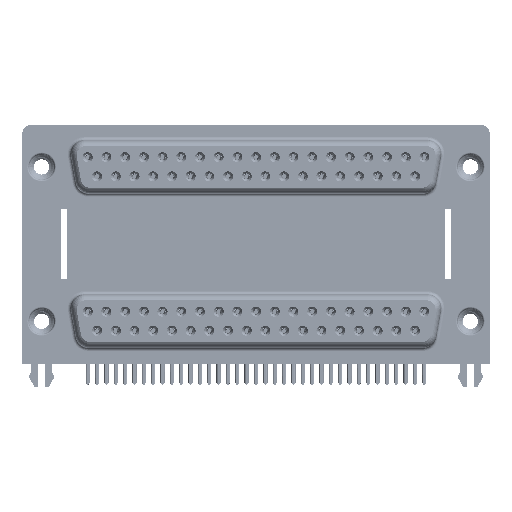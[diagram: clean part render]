
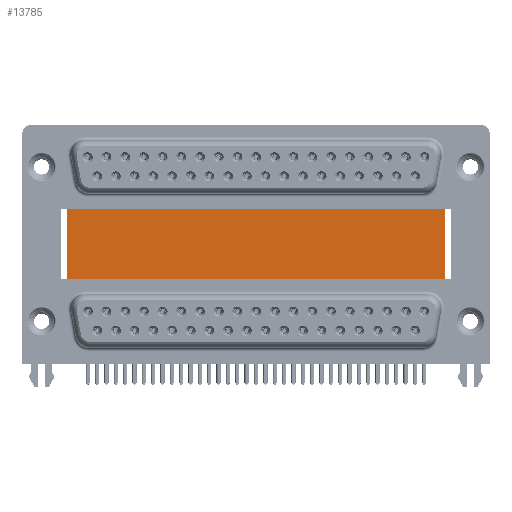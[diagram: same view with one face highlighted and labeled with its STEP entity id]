
A CAD part, top view. The second image highlights one B-rep face of the part: STEP entity #13785.
In plain terms, the highlighted planar face has unit normal (0, 0, 1).
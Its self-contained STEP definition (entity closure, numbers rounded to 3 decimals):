
#1719 = LINE ( 'NONE', #25269, #49968 ) ;
#2241 = PLANE ( 'NONE',  #61076 ) ;
#2263 = VECTOR ( 'NONE', #55672, 1000. ) ;
#5161 = VECTOR ( 'NONE', #67000, 1000. ) ;
#6648 = ORIENTED_EDGE ( 'NONE', *, *, #42072, .T. ) ;
#7897 = DIRECTION ( 'NONE',  ( 0., -1., 0. ) ) ;
#8912 = EDGE_CURVE ( 'NONE', #26235, #60179, #19910, .T. ) ;
#9746 = CARTESIAN_POINT ( 'NONE',  ( 59.71, 16.585, -12. ) ) ;
#12905 = ORIENTED_EDGE ( 'NONE', *, *, #69398, .F. ) ;
#13785 = ADVANCED_FACE ( 'NONE', ( #31564 ), #2241, .F. ) ;
#19817 = VERTEX_POINT ( 'NONE', #31889 ) ;
#19910 = LINE ( 'NONE', #43438, #5161 ) ;
#19995 = CARTESIAN_POINT ( 'NONE',  ( 3.79, 16.585, -12. ) ) ;
#20376 = ORIENTED_EDGE ( 'NONE', *, *, #32248, .F. ) ;
#20920 = CARTESIAN_POINT ( 'NONE',  ( 3.79, 16.585, -12. ) ) ;
#25269 = CARTESIAN_POINT ( 'NONE',  ( 3.79, 16.585, -12. ) ) ;
#26235 = VERTEX_POINT ( 'NONE', #37413 ) ;
#31170 = DIRECTION ( 'NONE',  ( -1., 0., 0. ) ) ;
#31564 = FACE_OUTER_BOUND ( 'NONE', #65779, .T. ) ;
#31889 = CARTESIAN_POINT ( 'NONE',  ( 59.71, 16.585, -12. ) ) ;
#32248 = EDGE_CURVE ( 'NONE', #19817, #60179, #57212, .T. ) ;
#32348 = CARTESIAN_POINT ( 'NONE',  ( 59.71, -3.735, -12. ) ) ;
#35272 = VECTOR ( 'NONE', #40453, 1000. ) ;
#37413 = CARTESIAN_POINT ( 'NONE',  ( 3.79, -3.735, -12. ) ) ;
#40453 = DIRECTION ( 'NONE',  ( 1., 0., 0. ) ) ;
#42072 = EDGE_CURVE ( 'NONE', #42598, #26235, #1719, .T. ) ;
#42598 = VERTEX_POINT ( 'NONE', #20920 ) ;
#43438 = CARTESIAN_POINT ( 'NONE',  ( 3.79, -3.735, -12. ) ) ;
#49968 = VECTOR ( 'NONE', #7897, 1000. ) ;
#51686 = CARTESIAN_POINT ( 'NONE',  ( 3.79, 16.585, -12. ) ) ;
#55672 = DIRECTION ( 'NONE',  ( 0., -1., 0. ) ) ;
#57212 = LINE ( 'NONE', #9746, #2263 ) ;
#60172 = DIRECTION ( 'NONE',  ( 0., 0., -1. ) ) ;
#60179 = VERTEX_POINT ( 'NONE', #32348 ) ;
#61076 = AXIS2_PLACEMENT_3D ( 'NONE', #19995, #60172, #31170 ) ;
#63403 = ORIENTED_EDGE ( 'NONE', *, *, #8912, .T. ) ;
#65779 = EDGE_LOOP ( 'NONE', ( #63403, #20376, #12905, #6648 ) ) ;
#67000 = DIRECTION ( 'NONE',  ( 1., 0., 0. ) ) ;
#69398 = EDGE_CURVE ( 'NONE', #42598, #19817, #74848, .T. ) ;
#74848 = LINE ( 'NONE', #51686, #35272 ) ;
